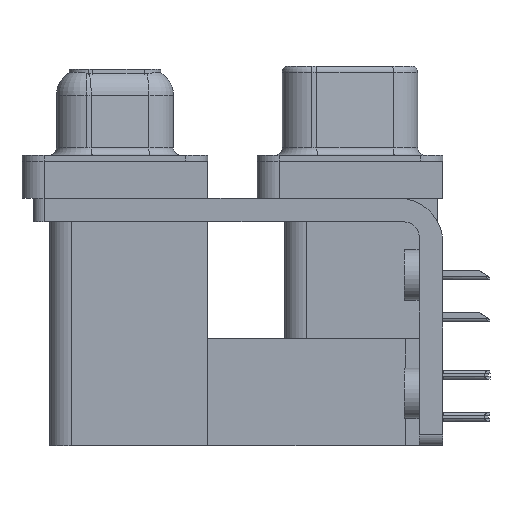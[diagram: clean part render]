
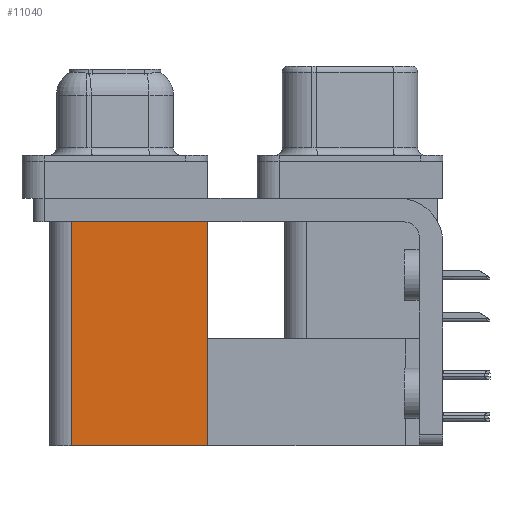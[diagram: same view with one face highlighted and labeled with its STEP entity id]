
A CAD part, left-side view. The second image highlights one B-rep face of the part: STEP entity #11040.
In plain terms, the highlighted planar face has unit normal (-1, 0, 0).
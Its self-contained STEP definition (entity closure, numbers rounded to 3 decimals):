
#639 = CARTESIAN_POINT ( 'NONE',  ( 3.765, 18.8, -19.2 ) ) ;
#759 = VERTEX_POINT ( 'NONE', #40305 ) ;
#1476 = VERTEX_POINT ( 'NONE', #6122 ) ;
#2924 = LINE ( 'NONE', #21245, #9817 ) ;
#3985 = CARTESIAN_POINT ( 'NONE',  ( 3.765, 9.6, -19.2 ) ) ;
#4252 = VECTOR ( 'NONE', #33451, 1000. ) ;
#5508 = ORIENTED_EDGE ( 'NONE', *, *, #42991, .F. ) ;
#6122 = CARTESIAN_POINT ( 'NONE',  ( 3.765, 18.8, -2.5 ) ) ;
#7529 = CARTESIAN_POINT ( 'NONE',  ( 3.765, 9.6, -19.2 ) ) ;
#9817 = VECTOR ( 'NONE', #16132, 1000. ) ;
#10458 = ORIENTED_EDGE ( 'NONE', *, *, #15620, .T. ) ;
#11040 = ADVANCED_FACE ( 'NONE', ( #40878 ), #40417, .F. ) ;
#11745 = DIRECTION ( 'NONE',  ( 0., 0., -1. ) ) ;
#12009 = CARTESIAN_POINT ( 'NONE',  ( 3.765, 9.6, -2.5 ) ) ;
#12866 = VERTEX_POINT ( 'NONE', #7529 ) ;
#15549 = CARTESIAN_POINT ( 'NONE',  ( 3.765, 9.6, -2.5 ) ) ;
#15620 = EDGE_CURVE ( 'NONE', #12866, #17213, #18425, .T. ) ;
#16132 = DIRECTION ( 'NONE',  ( 0., 1., 0. ) ) ;
#17213 = VERTEX_POINT ( 'NONE', #12009 ) ;
#18425 = LINE ( 'NONE', #18658, #4252 ) ;
#18491 = LINE ( 'NONE', #639, #36873 ) ;
#18658 = CARTESIAN_POINT ( 'NONE',  ( 3.765, 9.6, -19.2 ) ) ;
#18930 = DIRECTION ( 'NONE',  ( 0., 0., 1. ) ) ;
#19205 = VECTOR ( 'NONE', #45080, 1000. ) ;
#19871 = EDGE_LOOP ( 'NONE', ( #32917, #5508, #21544, #10458 ) ) ;
#21245 = CARTESIAN_POINT ( 'NONE',  ( 3.765, 9.6, -19.2 ) ) ;
#21544 = ORIENTED_EDGE ( 'NONE', *, *, #40232, .F. ) ;
#22826 = EDGE_CURVE ( 'NONE', #17213, #1476, #36914, .T. ) ;
#28104 = AXIS2_PLACEMENT_3D ( 'NONE', #3985, #29582, #11745 ) ;
#29582 = DIRECTION ( 'NONE',  ( 1., 0., 0. ) ) ;
#32917 = ORIENTED_EDGE ( 'NONE', *, *, #22826, .T. ) ;
#33451 = DIRECTION ( 'NONE',  ( 0., 0., 1. ) ) ;
#36873 = VECTOR ( 'NONE', #18930, 1000. ) ;
#36914 = LINE ( 'NONE', #15549, #19205 ) ;
#40232 = EDGE_CURVE ( 'NONE', #12866, #759, #2924, .T. ) ;
#40305 = CARTESIAN_POINT ( 'NONE',  ( 3.765, 18.8, -19.2 ) ) ;
#40417 = PLANE ( 'NONE',  #28104 ) ;
#40878 = FACE_OUTER_BOUND ( 'NONE', #19871, .T. ) ;
#42991 = EDGE_CURVE ( 'NONE', #759, #1476, #18491, .T. ) ;
#45080 = DIRECTION ( 'NONE',  ( 0., 1., 0. ) ) ;
